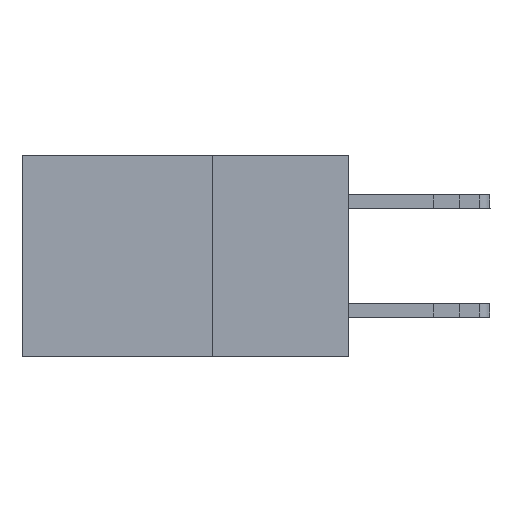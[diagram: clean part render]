
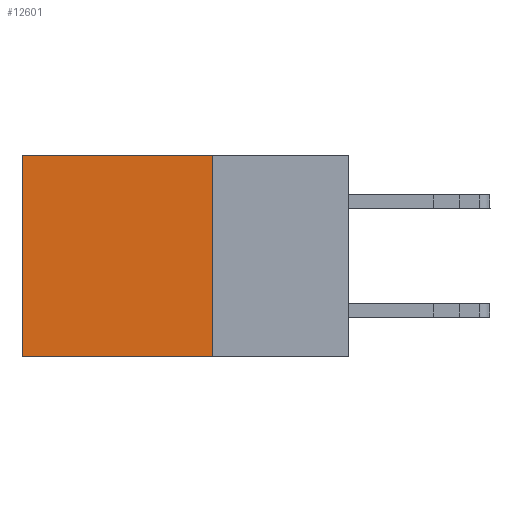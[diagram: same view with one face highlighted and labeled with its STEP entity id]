
A CAD part, left-side view. The second image highlights one B-rep face of the part: STEP entity #12601.
In plain terms, the highlighted planar face has unit normal (-1, 0, 0).
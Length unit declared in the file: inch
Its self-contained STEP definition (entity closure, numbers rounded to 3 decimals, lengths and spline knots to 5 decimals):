
#1019 = CARTESIAN_POINT ( 'NONE',  ( 0.298, 0.25, -0.37 ) ) ;
#1518 = CARTESIAN_POINT ( 'NONE',  ( 0.298, 0.6, -0.37 ) ) ;
#2105 = CARTESIAN_POINT ( 'NONE',  ( 0.298, 0.25, 0. ) ) ;
#4159 = ORIENTED_EDGE ( 'NONE', *, *, #14264, .T. ) ;
#4700 = ORIENTED_EDGE ( 'NONE', *, *, #5975, .F. ) ;
#5090 = VECTOR ( 'NONE', #19666, 39.37008 ) ;
#5975 = EDGE_CURVE ( 'NONE', #12725, #13284, #7143, .T. ) ;
#6135 = DIRECTION ( 'NONE',  ( 0., 1., 0. ) ) ;
#7131 = AXIS2_PLACEMENT_3D ( 'NONE', #2105, #22010, #9311 ) ;
#7143 = LINE ( 'NONE', #23096, #11099 ) ;
#7281 = CARTESIAN_POINT ( 'NONE',  ( 0.298, 0.6, 0. ) ) ;
#7362 = DIRECTION ( 'NONE',  ( 0., 0., -1. ) ) ;
#9170 = ORIENTED_EDGE ( 'NONE', *, *, #12777, .F. ) ;
#9311 = DIRECTION ( 'NONE',  ( 0., 0., -1. ) ) ;
#9580 = EDGE_LOOP ( 'NONE', ( #12710, #9170, #4700, #4159 ) ) ;
#10470 = VECTOR ( 'NONE', #7362, 39.37008 ) ;
#10674 = LINE ( 'NONE', #1019, #15460 ) ;
#11099 = VECTOR ( 'NONE', #14057, 39.37008 ) ;
#11500 = FACE_OUTER_BOUND ( 'NONE', #9580, .T. ) ;
#11868 = VERTEX_POINT ( 'NONE', #1518 ) ;
#12601 = ADVANCED_FACE ( 'NONE', ( #11500 ), #18509, .F. ) ;
#12710 = ORIENTED_EDGE ( 'NONE', *, *, #20641, .T. ) ;
#12725 = VERTEX_POINT ( 'NONE', #13686 ) ;
#12777 = EDGE_CURVE ( 'NONE', #13284, #11868, #10674, .T. ) ;
#13263 = LINE ( 'NONE', #7281, #10470 ) ;
#13284 = VERTEX_POINT ( 'NONE', #18404 ) ;
#13686 = CARTESIAN_POINT ( 'NONE',  ( 0.298, 0.25, 0. ) ) ;
#14057 = DIRECTION ( 'NONE',  ( 0., 0., -1. ) ) ;
#14264 = EDGE_CURVE ( 'NONE', #12725, #15070, #17572, .T. ) ;
#15070 = VERTEX_POINT ( 'NONE', #18042 ) ;
#15460 = VECTOR ( 'NONE', #6135, 39.37008 ) ;
#17572 = LINE ( 'NONE', #17840, #5090 ) ;
#17840 = CARTESIAN_POINT ( 'NONE',  ( 0.298, 0.25, 0. ) ) ;
#18042 = CARTESIAN_POINT ( 'NONE',  ( 0.298, 0.6, 0. ) ) ;
#18404 = CARTESIAN_POINT ( 'NONE',  ( 0.298, 0.25, -0.37 ) ) ;
#18509 = PLANE ( 'NONE',  #7131 ) ;
#19666 = DIRECTION ( 'NONE',  ( 0., 1., 0. ) ) ;
#20641 = EDGE_CURVE ( 'NONE', #15070, #11868, #13263, .T. ) ;
#22010 = DIRECTION ( 'NONE',  ( 1., 0., 0. ) ) ;
#23096 = CARTESIAN_POINT ( 'NONE',  ( 0.298, 0.25, 0. ) ) ;
